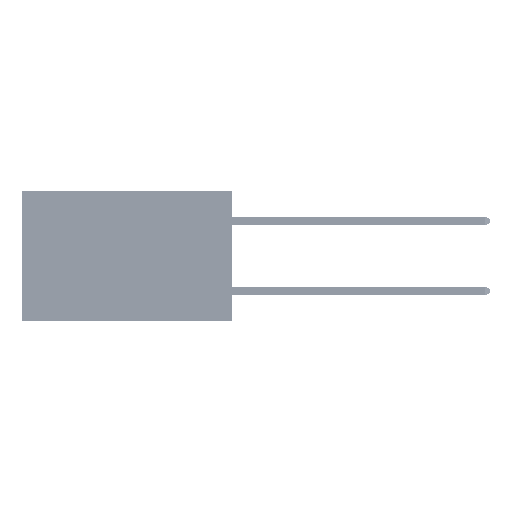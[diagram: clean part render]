
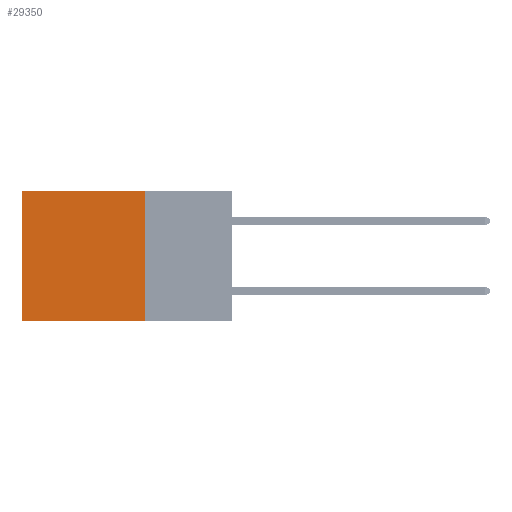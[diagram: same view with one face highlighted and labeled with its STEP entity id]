
A CAD part, left-side view. The second image highlights one B-rep face of the part: STEP entity #29350.
In plain terms, the highlighted planar face has unit normal (-1, 0, 0).
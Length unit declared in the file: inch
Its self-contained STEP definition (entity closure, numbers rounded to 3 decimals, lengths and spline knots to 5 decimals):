
#780 = CARTESIAN_POINT ( 'NONE',  ( 0.2875, 0.6, 0. ) ) ;
#960 = LINE ( 'NONE', #15872, #40058 ) ;
#2770 = CARTESIAN_POINT ( 'NONE',  ( 0.2875, 0.25, 0. ) ) ;
#3544 = LINE ( 'NONE', #10285, #22241 ) ;
#5732 = VERTEX_POINT ( 'NONE', #780 ) ;
#6760 = PLANE ( 'NONE',  #25613 ) ;
#10285 = CARTESIAN_POINT ( 'NONE',  ( 0.2875, 0.6, 0. ) ) ;
#10429 = CARTESIAN_POINT ( 'NONE',  ( 0.2875, 0.25, 0. ) ) ;
#11638 = DIRECTION ( 'NONE',  ( 0., 0., -1. ) ) ;
#14860 = CARTESIAN_POINT ( 'NONE',  ( 0.2875, 0.25, 0. ) ) ;
#14975 = DIRECTION ( 'NONE',  ( 0., 0., -1. ) ) ;
#15032 = VERTEX_POINT ( 'NONE', #35291 ) ;
#15630 = DIRECTION ( 'NONE',  ( 0., 1., 0. ) ) ;
#15872 = CARTESIAN_POINT ( 'NONE',  ( 0.2875, 0.25, -0.37 ) ) ;
#15985 = CARTESIAN_POINT ( 'NONE',  ( 0.2875, 0.25, 0. ) ) ;
#20937 = ORIENTED_EDGE ( 'NONE', *, *, #26616, .F. ) ;
#21894 = DIRECTION ( 'NONE',  ( 1., 0., 0. ) ) ;
#22241 = VECTOR ( 'NONE', #14975, 39.37008 ) ;
#25307 = VECTOR ( 'NONE', #11638, 39.37008 ) ;
#25613 = AXIS2_PLACEMENT_3D ( 'NONE', #2770, #21894, #37037 ) ;
#26039 = LINE ( 'NONE', #14860, #25307 ) ;
#26616 = EDGE_CURVE ( 'NONE', #30245, #43752, #26039, .T. ) ;
#26929 = ORIENTED_EDGE ( 'NONE', *, *, #29763, .T. ) ;
#29350 = ADVANCED_FACE ( 'NONE', ( #37769 ), #6760, .F. ) ;
#29763 = EDGE_CURVE ( 'NONE', #30245, #5732, #33757, .T. ) ;
#30032 = CARTESIAN_POINT ( 'NONE',  ( 0.2875, 0.25, -0.37 ) ) ;
#30245 = VERTEX_POINT ( 'NONE', #15985 ) ;
#33757 = LINE ( 'NONE', #10429, #35157 ) ;
#35157 = VECTOR ( 'NONE', #40460, 39.37008 ) ;
#35291 = CARTESIAN_POINT ( 'NONE',  ( 0.2875, 0.6, -0.37 ) ) ;
#37037 = DIRECTION ( 'NONE',  ( 0., 0., -1. ) ) ;
#37111 = ORIENTED_EDGE ( 'NONE', *, *, #39908, .T. ) ;
#37577 = EDGE_CURVE ( 'NONE', #43752, #15032, #960, .T. ) ;
#37769 = FACE_OUTER_BOUND ( 'NONE', #43103, .T. ) ;
#39908 = EDGE_CURVE ( 'NONE', #5732, #15032, #3544, .T. ) ;
#40058 = VECTOR ( 'NONE', #15630, 39.37008 ) ;
#40460 = DIRECTION ( 'NONE',  ( 0., 1., 0. ) ) ;
#43103 = EDGE_LOOP ( 'NONE', ( #37111, #47775, #20937, #26929 ) ) ;
#43752 = VERTEX_POINT ( 'NONE', #30032 ) ;
#47775 = ORIENTED_EDGE ( 'NONE', *, *, #37577, .F. ) ;
